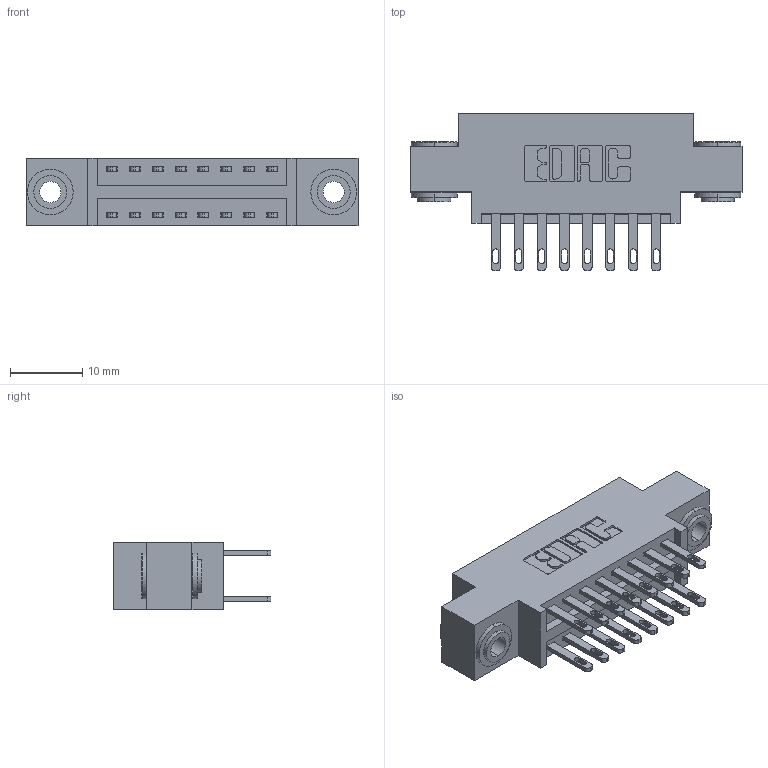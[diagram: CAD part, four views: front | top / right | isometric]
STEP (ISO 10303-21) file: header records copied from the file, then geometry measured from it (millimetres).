
FILE_DESCRIPTION (( 'STEP AP203' ), '1' );
FILE_NAME ('896-016-500-803.STEP', '2021-07-27T15:46:26', ( '' ), ( '' ), 'SwSTEP 2.0', 'SolidWorks 2020', '' );
FILE_SCHEMA (( 'CONFIG_CONTROL_DESIGN' ));
Length unit declared in the file: inch
Products named in the file (4): 896-016-500-803; 345-292-001_345-293-100; 846 Part_0.170 Offset - 0.156 Dia-TH; 345-250-002_345-250-002-102
Assembly tree (19 placements, depth 2):
  896-016-500-803
    846 Part_0.170 Offset - 0.156 Dia-TH
    345-292-001_345-293-100  x16
    345-250-002_345-250-002-102  x2
Bounding box: 45.97 x 21.84 x 9.4 mm (x, y, z)
Volume: 4132.6 mm3; surface area: 5707.5 mm2
Topology: 19 solids, 19 shells, 932 faces, 2769 edges, 1842 vertices
Faces by surface type: plane 554, cylinder 370, cone 8
Entity records: 10510 total; most frequent: CARTESIAN_POINT 1755, ORIENTED_EDGE 1682, DIRECTION 1631, EDGE_CURVE 841, VECTOR 649, LINE 649, VERTEX_POINT 558, AXIS2_PLACEMENT_3D 491
